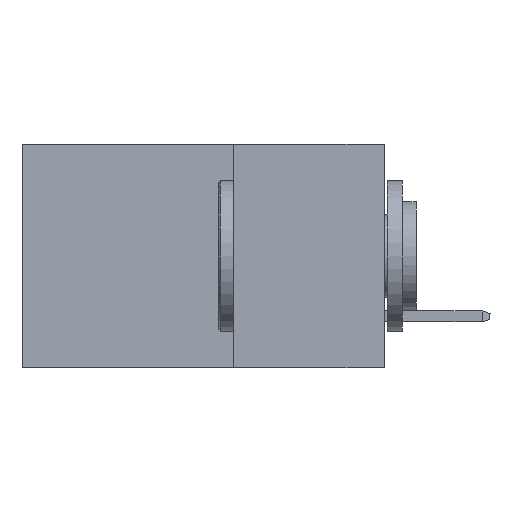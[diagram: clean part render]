
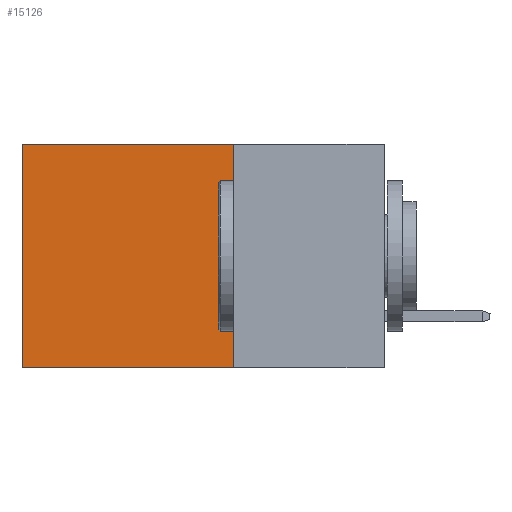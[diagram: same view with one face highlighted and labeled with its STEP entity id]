
A CAD part, left-side view. The second image highlights one B-rep face of the part: STEP entity #15126.
In plain terms, the highlighted planar face has unit normal (-1, 0, 0).
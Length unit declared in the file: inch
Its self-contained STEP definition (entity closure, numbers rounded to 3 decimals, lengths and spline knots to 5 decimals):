
#320 = DIRECTION ( 'NONE',  ( 0., 1., 0. ) ) ;
#1355 = ORIENTED_EDGE ( 'NONE', *, *, #6019, .T. ) ;
#1716 = CARTESIAN_POINT ( 'NONE',  ( 0.2615, 0.25, -0.37 ) ) ;
#2092 = VECTOR ( 'NONE', #3201, 39.37008 ) ;
#3201 = DIRECTION ( 'NONE',  ( 0., 0., -1. ) ) ;
#3824 = VERTEX_POINT ( 'NONE', #11980 ) ;
#5626 = CARTESIAN_POINT ( 'NONE',  ( 0.2615, 0.25, -0.37 ) ) ;
#5875 = FACE_OUTER_BOUND ( 'NONE', #5971, .T. ) ;
#5971 = EDGE_LOOP ( 'NONE', ( #1355, #7814, #21559, #23279 ) ) ;
#6019 = EDGE_CURVE ( 'NONE', #3824, #24759, #19219, .T. ) ;
#6460 = VECTOR ( 'NONE', #9571, 39.37008 ) ;
#7389 = DIRECTION ( 'NONE',  ( 0., 1., 0. ) ) ;
#7814 = ORIENTED_EDGE ( 'NONE', *, *, #22038, .F. ) ;
#8712 = LINE ( 'NONE', #16568, #25258 ) ;
#9429 = EDGE_CURVE ( 'NONE', #21500, #14062, #14678, .T. ) ;
#9571 = DIRECTION ( 'NONE',  ( 0., 0., -1. ) ) ;
#9626 = DIRECTION ( 'NONE',  ( 1., 0., 0. ) ) ;
#10801 = CARTESIAN_POINT ( 'NONE',  ( 0.2615, 0.25, -0.37 ) ) ;
#11421 = PLANE ( 'NONE',  #14813 ) ;
#11980 = CARTESIAN_POINT ( 'NONE',  ( 0.2615, 0.6, 0. ) ) ;
#14062 = VERTEX_POINT ( 'NONE', #22592 ) ;
#14678 = LINE ( 'NONE', #10801, #2092 ) ;
#14813 = AXIS2_PLACEMENT_3D ( 'NONE', #5626, #9626, #19272 ) ;
#15126 = ADVANCED_FACE ( 'NONE', ( #5875 ), #11421, .F. ) ;
#16568 = CARTESIAN_POINT ( 'NONE',  ( 0.2615, 0.25, 0. ) ) ;
#17070 = LINE ( 'NONE', #1716, #20278 ) ;
#19219 = LINE ( 'NONE', #19477, #6460 ) ;
#19272 = DIRECTION ( 'NONE',  ( 0., 0., -1. ) ) ;
#19477 = CARTESIAN_POINT ( 'NONE',  ( 0.2615, 0.6, -0.37 ) ) ;
#20278 = VECTOR ( 'NONE', #7389, 39.37008 ) ;
#21218 = CARTESIAN_POINT ( 'NONE',  ( 0.2615, 0.6, -0.37 ) ) ;
#21500 = VERTEX_POINT ( 'NONE', #24618 ) ;
#21559 = ORIENTED_EDGE ( 'NONE', *, *, #9429, .F. ) ;
#22038 = EDGE_CURVE ( 'NONE', #14062, #24759, #17070, .T. ) ;
#22592 = CARTESIAN_POINT ( 'NONE',  ( 0.2615, 0.25, -0.37 ) ) ;
#23279 = ORIENTED_EDGE ( 'NONE', *, *, #25059, .T. ) ;
#24618 = CARTESIAN_POINT ( 'NONE',  ( 0.2615, 0.25, 0. ) ) ;
#24759 = VERTEX_POINT ( 'NONE', #21218 ) ;
#25059 = EDGE_CURVE ( 'NONE', #21500, #3824, #8712, .T. ) ;
#25258 = VECTOR ( 'NONE', #320, 39.37008 ) ;
